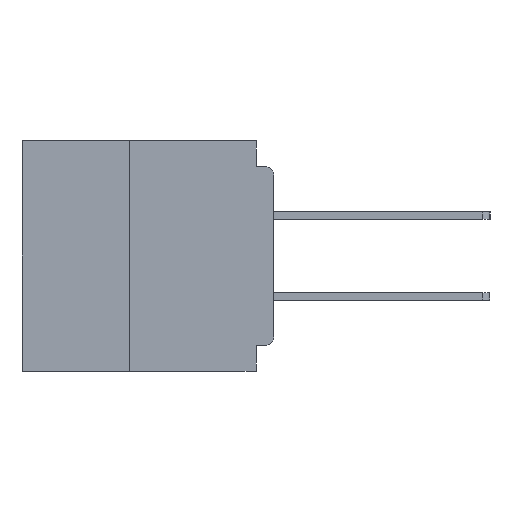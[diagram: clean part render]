
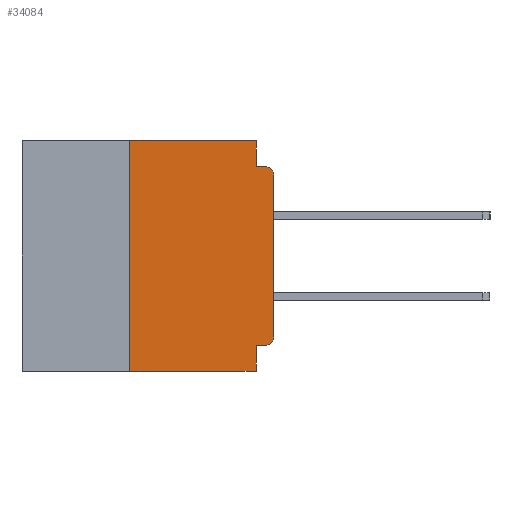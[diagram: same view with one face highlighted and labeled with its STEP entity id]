
A CAD part, left-side view. The second image highlights one B-rep face of the part: STEP entity #34084.
In plain terms, the highlighted planar face has unit normal (-1, 0, 0).
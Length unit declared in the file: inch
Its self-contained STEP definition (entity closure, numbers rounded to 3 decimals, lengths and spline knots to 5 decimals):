
#4080 = CIRCLE ( 'NONE', #19503, 0.015 ) ;
#5140 = CARTESIAN_POINT ( 'NONE',  ( 0., 0.031, 0. ) ) ;
#5874 = VECTOR ( 'NONE', #36082, 39.37008 ) ;
#6004 = VERTEX_POINT ( 'NONE', #53127 ) ;
#6845 = VECTOR ( 'NONE', #20570, 39.37008 ) ;
#8568 = DIRECTION ( 'NONE',  ( 0., 0., -1. ) ) ;
#9891 = EDGE_CURVE ( 'NONE', #66322, #32950, #53151, .T. ) ;
#10098 = VERTEX_POINT ( 'NONE', #5140 ) ;
#10318 = LINE ( 'NONE', #20209, #50191 ) ;
#13372 = ORIENTED_EDGE ( 'NONE', *, *, #9891, .F. ) ;
#14463 = EDGE_CURVE ( 'NONE', #16427, #32950, #19669, .T. ) ;
#15243 = DIRECTION ( 'NONE',  ( 0., -1., 0. ) ) ;
#16195 = DIRECTION ( 'NONE',  ( 0., -1., 0. ) ) ;
#16427 = VERTEX_POINT ( 'NONE', #40666 ) ;
#16541 = AXIS2_PLACEMENT_3D ( 'NONE', #48931, #17732, #54139 ) ;
#16673 = CARTESIAN_POINT ( 'NONE',  ( 0., 0.015, -0.355 ) ) ;
#17732 = DIRECTION ( 'NONE',  ( -1., 0., 0. ) ) ;
#19503 = AXIS2_PLACEMENT_3D ( 'NONE', #24315, #60784, #29558 ) ;
#19669 = LINE ( 'NONE', #42873, #59639 ) ;
#20209 = CARTESIAN_POINT ( 'NONE',  ( 0., 0., -0.045 ) ) ;
#20570 = DIRECTION ( 'NONE',  ( 0., 0., 1. ) ) ;
#21149 = CARTESIAN_POINT ( 'NONE',  ( 0., 0.437, 0. ) ) ;
#22703 = ORIENTED_EDGE ( 'NONE', *, *, #25315, .F. ) ;
#24152 = VECTOR ( 'NONE', #16195, 39.37008 ) ;
#24315 = CARTESIAN_POINT ( 'NONE',  ( 0., 0.015, -0.34 ) ) ;
#24651 = CARTESIAN_POINT ( 'NONE',  ( 0., 0.031, -0.4 ) ) ;
#25208 = FACE_OUTER_BOUND ( 'NONE', #26656, .T. ) ;
#25315 = EDGE_CURVE ( 'NONE', #16427, #35672, #29685, .T. ) ;
#25407 = VECTOR ( 'NONE', #66293, 39.37008 ) ;
#25823 = CARTESIAN_POINT ( 'NONE',  ( 0., 0., 0. ) ) ;
#26234 = ORIENTED_EDGE ( 'NONE', *, *, #48020, .T. ) ;
#26656 = EDGE_LOOP ( 'NONE', ( #54113, #35380, #54910, #46912, #62310, #22703, #35198, #13372, #28413, #26234 ) ) ;
#27067 = CARTESIAN_POINT ( 'NONE',  ( 0., 0.25, 0. ) ) ;
#27695 = VERTEX_POINT ( 'NONE', #16673 ) ;
#28413 = ORIENTED_EDGE ( 'NONE', *, *, #40020, .F. ) ;
#29558 = DIRECTION ( 'NONE',  ( 0., 0., -1. ) ) ;
#29685 = LINE ( 'NONE', #63139, #55782 ) ;
#30847 = CARTESIAN_POINT ( 'NONE',  ( 0., 0., -0.355 ) ) ;
#32950 = VERTEX_POINT ( 'NONE', #61477 ) ;
#33058 = VERTEX_POINT ( 'NONE', #62579 ) ;
#33492 = LINE ( 'NONE', #30847, #5874 ) ;
#34084 = ADVANCED_FACE ( 'NONE', ( #25208 ), #34439, .F. ) ;
#34439 = PLANE ( 'NONE',  #47060 ) ;
#34682 = EDGE_CURVE ( 'NONE', #10098, #33058, #37060, .T. ) ;
#35198 = ORIENTED_EDGE ( 'NONE', *, *, #14463, .T. ) ;
#35380 = ORIENTED_EDGE ( 'NONE', *, *, #39709, .T. ) ;
#35577 = EDGE_CURVE ( 'NONE', #35672, #10098, #38051, .T. ) ;
#35672 = VERTEX_POINT ( 'NONE', #27067 ) ;
#36037 = EDGE_CURVE ( 'NONE', #33058, #6004, #10318, .T. ) ;
#36082 = DIRECTION ( 'NONE',  ( 0., 1., 0. ) ) ;
#37060 = LINE ( 'NONE', #45778, #39811 ) ;
#38051 = LINE ( 'NONE', #21149, #24152 ) ;
#38208 = EDGE_CURVE ( 'NONE', #44228, #65681, #63798, .T. ) ;
#39702 = DIRECTION ( 'NONE',  ( 1., 0., 0. ) ) ;
#39709 = EDGE_CURVE ( 'NONE', #65681, #6004, #54744, .T. ) ;
#39811 = VECTOR ( 'NONE', #56243, 39.37008 ) ;
#40020 = EDGE_CURVE ( 'NONE', #27695, #66322, #33492, .T. ) ;
#40666 = CARTESIAN_POINT ( 'NONE',  ( 0., 0.25, -0.4 ) ) ;
#42873 = CARTESIAN_POINT ( 'NONE',  ( 0., 0.437, -0.4 ) ) ;
#44121 = CARTESIAN_POINT ( 'NONE',  ( 0., 0.031, -0.355 ) ) ;
#44228 = VERTEX_POINT ( 'NONE', #64085 ) ;
#45778 = CARTESIAN_POINT ( 'NONE',  ( 0., 0.031, 0. ) ) ;
#46912 = ORIENTED_EDGE ( 'NONE', *, *, #34682, .F. ) ;
#47060 = AXIS2_PLACEMENT_3D ( 'NONE', #65602, #39702, #8568 ) ;
#47697 = DIRECTION ( 'NONE',  ( 0., 0., 1. ) ) ;
#48020 = EDGE_CURVE ( 'NONE', #27695, #44228, #4080, .T. ) ;
#48931 = CARTESIAN_POINT ( 'NONE',  ( 0., 0.015, -0.06 ) ) ;
#50191 = VECTOR ( 'NONE', #15243, 39.37008 ) ;
#53127 = CARTESIAN_POINT ( 'NONE',  ( 0., 0.015, -0.045 ) ) ;
#53151 = LINE ( 'NONE', #24651, #25407 ) ;
#54113 = ORIENTED_EDGE ( 'NONE', *, *, #38208, .T. ) ;
#54139 = DIRECTION ( 'NONE',  ( 0., 0., -1. ) ) ;
#54744 = CIRCLE ( 'NONE', #16541, 0.015 ) ;
#54910 = ORIENTED_EDGE ( 'NONE', *, *, #36037, .F. ) ;
#55782 = VECTOR ( 'NONE', #47697, 39.37008 ) ;
#56243 = DIRECTION ( 'NONE',  ( 0., 0., -1. ) ) ;
#58618 = DIRECTION ( 'NONE',  ( 0., -1., 0. ) ) ;
#59639 = VECTOR ( 'NONE', #58618, 39.37008 ) ;
#60784 = DIRECTION ( 'NONE',  ( -1., 0., 0. ) ) ;
#61477 = CARTESIAN_POINT ( 'NONE',  ( 0., 0.031, -0.4 ) ) ;
#62310 = ORIENTED_EDGE ( 'NONE', *, *, #35577, .F. ) ;
#62579 = CARTESIAN_POINT ( 'NONE',  ( 0., 0.031, -0.045 ) ) ;
#63139 = CARTESIAN_POINT ( 'NONE',  ( 0., 0.25, -0.4 ) ) ;
#63798 = LINE ( 'NONE', #25823, #6845 ) ;
#64085 = CARTESIAN_POINT ( 'NONE',  ( 0., 0., -0.34 ) ) ;
#64669 = CARTESIAN_POINT ( 'NONE',  ( 0., 0., -0.06 ) ) ;
#65602 = CARTESIAN_POINT ( 'NONE',  ( 0., 0.437, 0. ) ) ;
#65681 = VERTEX_POINT ( 'NONE', #64669 ) ;
#66293 = DIRECTION ( 'NONE',  ( 0., 0., -1. ) ) ;
#66322 = VERTEX_POINT ( 'NONE', #44121 ) ;
